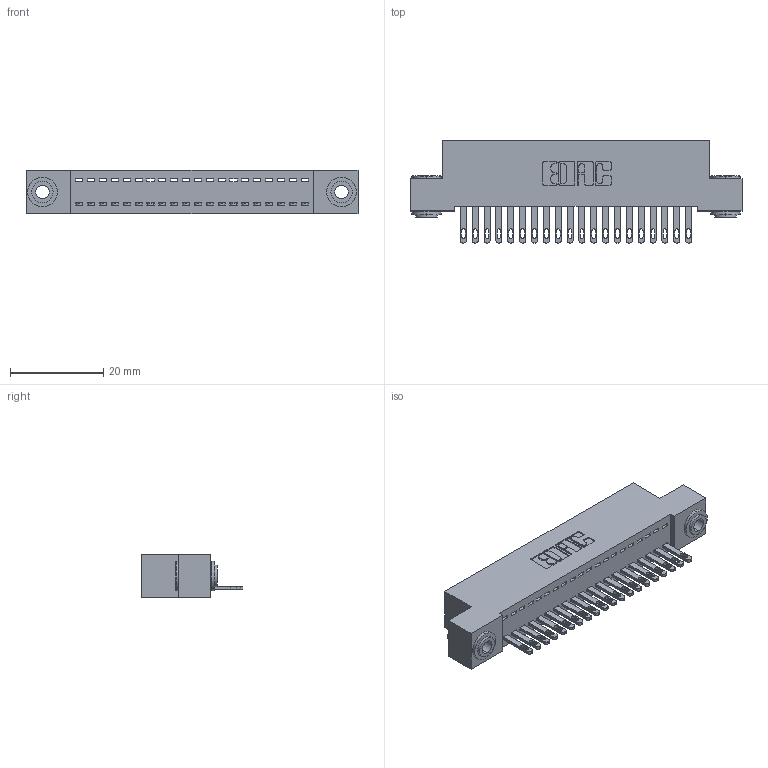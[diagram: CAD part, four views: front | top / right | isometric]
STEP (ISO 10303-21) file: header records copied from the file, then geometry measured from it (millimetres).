
FILE_DESCRIPTION (( 'STEP AP203' ), '1' );
FILE_NAME ('892-020-500-103.STEP', '2020-09-21T13:52:57', ( '' ), ( '' ), 'SwSTEP 2.0', 'SolidWorks 2020', '' );
FILE_SCHEMA (( 'CONFIG_CONTROL_DESIGN' ));
Length unit declared in the file: inch
Products named in the file (4): 345-292-001_345-293-100; 342-250-002_345-250-002-102; 892-020-500-103; 842 Part_.156 TH
Assembly tree (23 placements, depth 2):
  892-020-500-103
    842 Part_.156 TH
    345-292-001_345-293-100  x20
    342-250-002_345-250-002-102  x2
Bounding box: 71.12 x 21.85 x 9.4 mm (x, y, z)
Volume: 6190 mm3; surface area: 8944.4 mm2
Topology: 23 solids, 23 shells, 1228 faces, 3735 edges, 2486 vertices
Faces by surface type: plane 796, cylinder 424, cone 8
Entity records: 15520 total; most frequent: CARTESIAN_POINT 2657, ORIENTED_EDGE 2606, DIRECTION 2321, EDGE_CURVE 1303, VECTOR 1147, LINE 1147, VERTEX_POINT 866, AXIS2_PLACEMENT_3D 587
